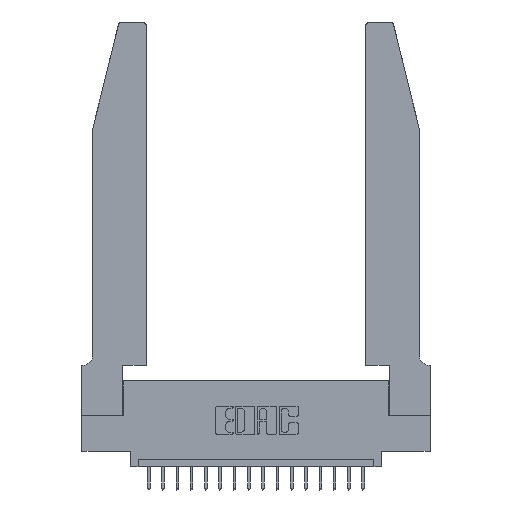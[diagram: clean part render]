
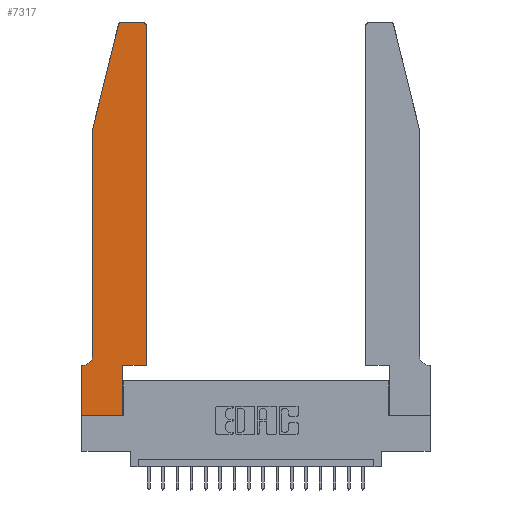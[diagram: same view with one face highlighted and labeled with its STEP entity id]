
A CAD part, top view. The second image highlights one B-rep face of the part: STEP entity #7317.
In plain terms, the highlighted planar face has unit normal (0, 0, 1).
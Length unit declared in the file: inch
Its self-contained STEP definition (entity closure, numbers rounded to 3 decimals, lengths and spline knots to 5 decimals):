
#96 = DIRECTION ( 'NONE',  ( 0., -1., 0. ) ) ;
#153 = LINE ( 'NONE', #6723, #14284 ) ;
#844 = VERTEX_POINT ( 'NONE', #20057 ) ;
#1139 = DIRECTION ( 'NONE',  ( -1., 0., 0. ) ) ;
#1549 = VECTOR ( 'NONE', #3644, 39.37008 ) ;
#1608 = ORIENTED_EDGE ( 'NONE', *, *, #6840, .T. ) ;
#1677 = CARTESIAN_POINT ( 'NONE',  ( 0., 0., 0.37 ) ) ;
#1852 = VECTOR ( 'NONE', #7059, 39.37008 ) ;
#2103 = EDGE_CURVE ( 'NONE', #20310, #19635, #7856, .T. ) ;
#2245 = ORIENTED_EDGE ( 'NONE', *, *, #2103, .T. ) ;
#2259 = LINE ( 'NONE', #8081, #20365 ) ;
#2304 = AXIS2_PLACEMENT_3D ( 'NONE', #14379, #14786, #10298 ) ;
#2400 = EDGE_CURVE ( 'NONE', #6962, #3588, #12771, .T. ) ;
#2731 = CARTESIAN_POINT ( 'NONE',  ( 0.2865, 0.35, 0.37 ) ) ;
#2769 = ORIENTED_EDGE ( 'NONE', *, *, #2400, .T. ) ;
#2995 = CIRCLE ( 'NONE', #3485, 0.03 ) ;
#3279 = LINE ( 'NONE', #11309, #1549 ) ;
#3485 = AXIS2_PLACEMENT_3D ( 'NONE', #16831, #8821, #9617 ) ;
#3588 = VERTEX_POINT ( 'NONE', #5794 ) ;
#3644 = DIRECTION ( 'NONE',  ( 0., 1., 0. ) ) ;
#4020 = VERTEX_POINT ( 'NONE', #2731 ) ;
#4822 = DIRECTION ( 'NONE',  ( 0., -1., 0. ) ) ;
#5121 = EDGE_CURVE ( 'NONE', #4020, #5544, #11508, .T. ) ;
#5207 = VERTEX_POINT ( 'NONE', #19059 ) ;
#5260 = ORIENTED_EDGE ( 'NONE', *, *, #13033, .T. ) ;
#5334 = VECTOR ( 'NONE', #96, 39.37008 ) ;
#5413 = EDGE_LOOP ( 'NONE', ( #13802, #2245, #14937, #6223, #9127, #7631, #2769, #7442, #5260, #19560, #8921, #1608 ) ) ;
#5441 = CARTESIAN_POINT ( 'NONE',  ( 0.0755, 2., 0.37 ) ) ;
#5544 = VERTEX_POINT ( 'NONE', #19845 ) ;
#5794 = CARTESIAN_POINT ( 'NONE',  ( 0., 0., 0.37 ) ) ;
#6223 = ORIENTED_EDGE ( 'NONE', *, *, #17842, .T. ) ;
#6485 = AXIS2_PLACEMENT_3D ( 'NONE', #13826, #9206, #1139 ) ;
#6524 = DIRECTION ( 'NONE',  ( 1., 0., 0. ) ) ;
#6706 = CARTESIAN_POINT ( 'NONE',  ( 0.2605, 2.75, 0.37 ) ) ;
#6723 = CARTESIAN_POINT ( 'NONE',  ( 0.0755, 0.35, 0.37 ) ) ;
#6840 = EDGE_CURVE ( 'NONE', #844, #17613, #2995, .T. ) ;
#6962 = VERTEX_POINT ( 'NONE', #15523 ) ;
#7059 = DIRECTION ( 'NONE',  ( 0., 1., 0. ) ) ;
#7317 = ADVANCED_FACE ( 'NONE', ( #10419 ), #15142, .T. ) ;
#7442 = ORIENTED_EDGE ( 'NONE', *, *, #11595, .T. ) ;
#7504 = CARTESIAN_POINT ( 'NONE',  ( 0.4505, 0.35, 0.37 ) ) ;
#7631 = ORIENTED_EDGE ( 'NONE', *, *, #17390, .T. ) ;
#7826 = VECTOR ( 'NONE', #13253, 39.37008 ) ;
#7856 = CIRCLE ( 'NONE', #14440, 0.03 ) ;
#8081 = CARTESIAN_POINT ( 'NONE',  ( 0.0755, 2., 0.37 ) ) ;
#8272 = VERTEX_POINT ( 'NONE', #13837 ) ;
#8674 = VECTOR ( 'NONE', #11146, 39.37008 ) ;
#8821 = DIRECTION ( 'NONE',  ( 0., 0., 1. ) ) ;
#8921 = ORIENTED_EDGE ( 'NONE', *, *, #10512, .T. ) ;
#9127 = ORIENTED_EDGE ( 'NONE', *, *, #18891, .T. ) ;
#9174 = CIRCLE ( 'NONE', #6485, 0.07 ) ;
#9206 = DIRECTION ( 'NONE',  ( 0., 0., -1. ) ) ;
#9413 = VECTOR ( 'NONE', #10246, 39.37008 ) ;
#9570 = LINE ( 'NONE', #11537, #7826 ) ;
#9617 = DIRECTION ( 'NONE',  ( 1., 0., 0. ) ) ;
#9917 = DIRECTION ( 'NONE',  ( -1., 0., 0. ) ) ;
#10246 = DIRECTION ( 'NONE',  ( -0.239, -0.971, 0. ) ) ;
#10298 = DIRECTION ( 'NONE',  ( 1., 0., 0. ) ) ;
#10382 = LINE ( 'NONE', #5441, #9413 ) ;
#10419 = FACE_OUTER_BOUND ( 'NONE', #5413, .T. ) ;
#10512 = EDGE_CURVE ( 'NONE', #5544, #844, #15471, .T. ) ;
#10574 = CARTESIAN_POINT ( 'NONE',  ( 0.0055, 0.35, 0.37 ) ) ;
#11146 = DIRECTION ( 'NONE',  ( -1., 0., 0. ) ) ;
#11309 = CARTESIAN_POINT ( 'NONE',  ( 0.2865, 0.35, 0.37 ) ) ;
#11508 = LINE ( 'NONE', #7504, #19435 ) ;
#11537 = CARTESIAN_POINT ( 'NONE',  ( 0., 0., 0.37 ) ) ;
#11595 = EDGE_CURVE ( 'NONE', #3588, #5207, #9570, .T. ) ;
#11758 = VERTEX_POINT ( 'NONE', #15439 ) ;
#11939 = CARTESIAN_POINT ( 'NONE',  ( 0.4205, 2.75, 0.37 ) ) ;
#12771 = LINE ( 'NONE', #1677, #5334 ) ;
#13033 = EDGE_CURVE ( 'NONE', #5207, #4020, #3279, .T. ) ;
#13194 = CARTESIAN_POINT ( 'NONE',  ( 0.284, 2.75, 0.37 ) ) ;
#13253 = DIRECTION ( 'NONE',  ( 1., 0., 0. ) ) ;
#13802 = ORIENTED_EDGE ( 'NONE', *, *, #14925, .T. ) ;
#13826 = CARTESIAN_POINT ( 'NONE',  ( 0.0055, 0.42, 0.37 ) ) ;
#13837 = CARTESIAN_POINT ( 'NONE',  ( 0.0755, 0.42, 0.37 ) ) ;
#14284 = VECTOR ( 'NONE', #9917, 39.37008 ) ;
#14379 = CARTESIAN_POINT ( 'NONE',  ( 0., 0.35, 0.37 ) ) ;
#14440 = AXIS2_PLACEMENT_3D ( 'NONE', #15515, #20221, #6524 ) ;
#14628 = LINE ( 'NONE', #6706, #8674 ) ;
#14786 = DIRECTION ( 'NONE',  ( 0., 0., 1. ) ) ;
#14925 = EDGE_CURVE ( 'NONE', #17613, #20310, #14628, .T. ) ;
#14937 = ORIENTED_EDGE ( 'NONE', *, *, #15803, .T. ) ;
#15142 = PLANE ( 'NONE',  #2304 ) ;
#15439 = CARTESIAN_POINT ( 'NONE',  ( 0.0755, 2., 0.37 ) ) ;
#15471 = LINE ( 'NONE', #18311, #1852 ) ;
#15515 = CARTESIAN_POINT ( 'NONE',  ( 0.284, 2.72, 0.37 ) ) ;
#15523 = CARTESIAN_POINT ( 'NONE',  ( 0., 0.35, 0.37 ) ) ;
#15803 = EDGE_CURVE ( 'NONE', #19635, #11758, #10382, .T. ) ;
#16831 = CARTESIAN_POINT ( 'NONE',  ( 0.4205, 2.72, 0.37 ) ) ;
#17390 = EDGE_CURVE ( 'NONE', #17597, #6962, #153, .T. ) ;
#17597 = VERTEX_POINT ( 'NONE', #10574 ) ;
#17613 = VERTEX_POINT ( 'NONE', #11939 ) ;
#17809 = CARTESIAN_POINT ( 'NONE',  ( 0.25487, 2.72718, 0.37 ) ) ;
#17842 = EDGE_CURVE ( 'NONE', #11758, #8272, #2259, .T. ) ;
#18311 = CARTESIAN_POINT ( 'NONE',  ( 0.4505, 0.35, 0.37 ) ) ;
#18782 = DIRECTION ( 'NONE',  ( 1., 0., 0. ) ) ;
#18891 = EDGE_CURVE ( 'NONE', #8272, #17597, #9174, .T. ) ;
#19059 = CARTESIAN_POINT ( 'NONE',  ( 0.2865, 0., 0.37 ) ) ;
#19435 = VECTOR ( 'NONE', #18782, 39.37008 ) ;
#19560 = ORIENTED_EDGE ( 'NONE', *, *, #5121, .T. ) ;
#19635 = VERTEX_POINT ( 'NONE', #17809 ) ;
#19845 = CARTESIAN_POINT ( 'NONE',  ( 0.4505, 0.35, 0.37 ) ) ;
#20057 = CARTESIAN_POINT ( 'NONE',  ( 0.4505, 2.72, 0.37 ) ) ;
#20221 = DIRECTION ( 'NONE',  ( 0., 0., 1. ) ) ;
#20310 = VERTEX_POINT ( 'NONE', #13194 ) ;
#20365 = VECTOR ( 'NONE', #4822, 39.37008 ) ;
